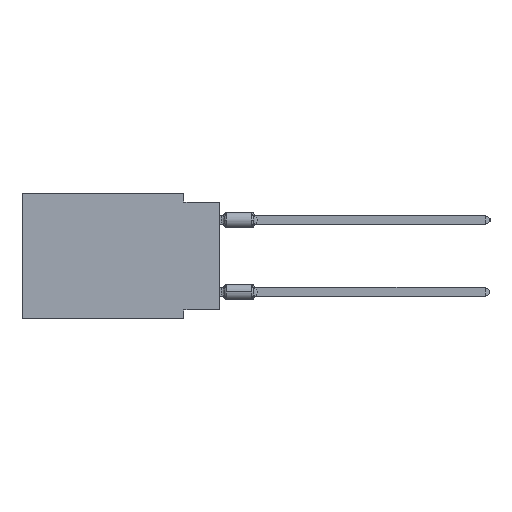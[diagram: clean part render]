
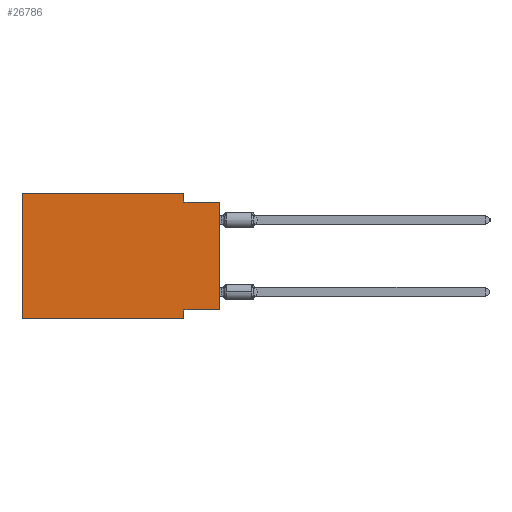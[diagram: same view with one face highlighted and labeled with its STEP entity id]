
A CAD part, left-side view. The second image highlights one B-rep face of the part: STEP entity #26786.
In plain terms, the highlighted planar face has unit normal (-1, 0, 0).
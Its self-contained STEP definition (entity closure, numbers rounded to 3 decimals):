
#251 = VECTOR ( 'NONE', #1010, 1000. ) ;
#978 = VERTEX_POINT ( 'NONE', #11297 ) ;
#1010 = DIRECTION ( 'NONE',  ( 0., -1., 0. ) ) ;
#2933 = LINE ( 'NONE', #44178, #10374 ) ;
#3685 = VERTEX_POINT ( 'NONE', #15809 ) ;
#4828 = LINE ( 'NONE', #42268, #251 ) ;
#5890 = CARTESIAN_POINT ( 'NONE',  ( 0., 0., 0. ) ) ;
#6622 = CARTESIAN_POINT ( 'NONE',  ( 0., 0., -8.255 ) ) ;
#7270 = EDGE_CURVE ( 'NONE', #18120, #3685, #48133, .T. ) ;
#7845 = LINE ( 'NONE', #52374, #38607 ) ;
#8441 = VERTEX_POINT ( 'NONE', #18316 ) ;
#8609 = ORIENTED_EDGE ( 'NONE', *, *, #26036, .F. ) ;
#9545 = DIRECTION ( 'NONE',  ( 0., 0., 1. ) ) ;
#9565 = VECTOR ( 'NONE', #44921, 1000. ) ;
#9613 = PLANE ( 'NONE',  #49246 ) ;
#9875 = ORIENTED_EDGE ( 'NONE', *, *, #23795, .F. ) ;
#10374 = VECTOR ( 'NONE', #35778, 1000. ) ;
#11297 = CARTESIAN_POINT ( 'NONE',  ( 0., 13.97, 0. ) ) ;
#11819 = LINE ( 'NONE', #28401, #9565 ) ;
#14224 = CARTESIAN_POINT ( 'NONE',  ( 0., 13.97, 0. ) ) ;
#14676 = VERTEX_POINT ( 'NONE', #47090 ) ;
#15364 = LINE ( 'NONE', #5890, #45984 ) ;
#15809 = CARTESIAN_POINT ( 'NONE',  ( 0., 2.54, -8.255 ) ) ;
#18120 = VERTEX_POINT ( 'NONE', #6622 ) ;
#18285 = VECTOR ( 'NONE', #21181, 1000. ) ;
#18316 = CARTESIAN_POINT ( 'NONE',  ( 0., 2.54, 0. ) ) ;
#18603 = CARTESIAN_POINT ( 'NONE',  ( 0., 2.54, -8.89 ) ) ;
#21169 = VECTOR ( 'NONE', #48396, 1000. ) ;
#21181 = DIRECTION ( 'NONE',  ( 0., -1., 0. ) ) ;
#23319 = VERTEX_POINT ( 'NONE', #18603 ) ;
#23795 = EDGE_CURVE ( 'NONE', #8441, #14676, #7845, .T. ) ;
#26036 = EDGE_CURVE ( 'NONE', #42896, #978, #30203, .T. ) ;
#26786 = ADVANCED_FACE ( 'NONE', ( #51399 ), #9613, .F. ) ;
#28226 = DIRECTION ( 'NONE',  ( 0., 0., -1. ) ) ;
#28401 = CARTESIAN_POINT ( 'NONE',  ( 0., 13.97, -8.89 ) ) ;
#28510 = EDGE_CURVE ( 'NONE', #978, #8441, #37996, .T. ) ;
#28865 = ORIENTED_EDGE ( 'NONE', *, *, #28510, .F. ) ;
#30203 = LINE ( 'NONE', #46720, #49181 ) ;
#30517 = EDGE_CURVE ( 'NONE', #14676, #43187, #4828, .T. ) ;
#30796 = DIRECTION ( 'NONE',  ( 1., 0., 0. ) ) ;
#32956 = ORIENTED_EDGE ( 'NONE', *, *, #30517, .F. ) ;
#33456 = ORIENTED_EDGE ( 'NONE', *, *, #39405, .T. ) ;
#33671 = CARTESIAN_POINT ( 'NONE',  ( 0., 13.97, 0. ) ) ;
#35778 = DIRECTION ( 'NONE',  ( 0., 0., -1. ) ) ;
#37996 = LINE ( 'NONE', #33671, #18285 ) ;
#38607 = VECTOR ( 'NONE', #28226, 1000. ) ;
#38778 = EDGE_CURVE ( 'NONE', #3685, #23319, #2933, .T. ) ;
#39155 = ORIENTED_EDGE ( 'NONE', *, *, #39195, .T. ) ;
#39195 = EDGE_CURVE ( 'NONE', #18120, #43187, #15364, .T. ) ;
#39405 = EDGE_CURVE ( 'NONE', #42896, #23319, #11819, .T. ) ;
#39441 = ORIENTED_EDGE ( 'NONE', *, *, #7270, .F. ) ;
#41071 = CARTESIAN_POINT ( 'NONE',  ( 0., 0., -8.255 ) ) ;
#42268 = CARTESIAN_POINT ( 'NONE',  ( 0., 0., -0.635 ) ) ;
#42277 = ORIENTED_EDGE ( 'NONE', *, *, #38778, .F. ) ;
#42896 = VERTEX_POINT ( 'NONE', #50755 ) ;
#43187 = VERTEX_POINT ( 'NONE', #45814 ) ;
#43868 = DIRECTION ( 'NONE',  ( 0., 0., 1. ) ) ;
#44178 = CARTESIAN_POINT ( 'NONE',  ( 0., 2.54, -8.89 ) ) ;
#44921 = DIRECTION ( 'NONE',  ( 0., -1., 0. ) ) ;
#45814 = CARTESIAN_POINT ( 'NONE',  ( 0., 0., -0.635 ) ) ;
#45984 = VECTOR ( 'NONE', #43868, 1000. ) ;
#46720 = CARTESIAN_POINT ( 'NONE',  ( 0., 13.97, 0. ) ) ;
#47090 = CARTESIAN_POINT ( 'NONE',  ( 0., 2.54, -0.635 ) ) ;
#47323 = DIRECTION ( 'NONE',  ( 0., 0., -1. ) ) ;
#48133 = LINE ( 'NONE', #41071, #21169 ) ;
#48396 = DIRECTION ( 'NONE',  ( 0., 1., 0. ) ) ;
#49181 = VECTOR ( 'NONE', #9545, 1000. ) ;
#49246 = AXIS2_PLACEMENT_3D ( 'NONE', #14224, #30796, #47323 ) ;
#49291 = EDGE_LOOP ( 'NONE', ( #39155, #32956, #9875, #28865, #8609, #33456, #42277, #39441 ) ) ;
#50755 = CARTESIAN_POINT ( 'NONE',  ( 0., 13.97, -8.89 ) ) ;
#51399 = FACE_OUTER_BOUND ( 'NONE', #49291, .T. ) ;
#52374 = CARTESIAN_POINT ( 'NONE',  ( 0., 2.54, 0. ) ) ;
